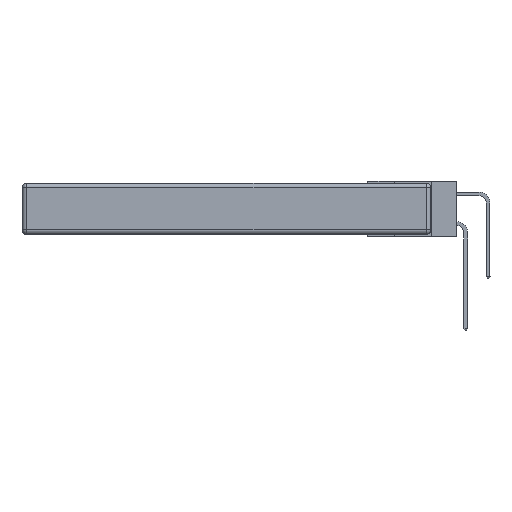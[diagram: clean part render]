
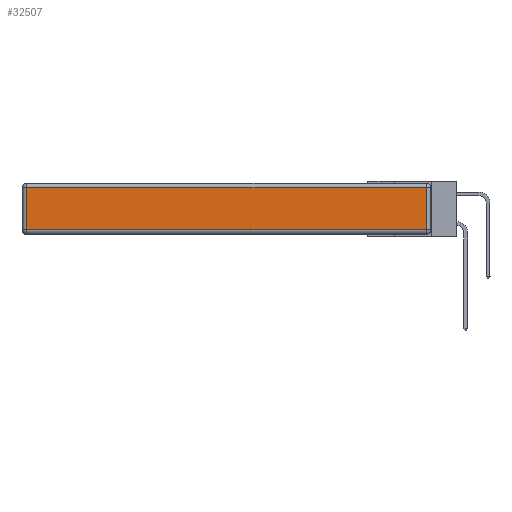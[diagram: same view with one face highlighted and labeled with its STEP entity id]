
A CAD part, left-side view. The second image highlights one B-rep face of the part: STEP entity #32507.
In plain terms, the highlighted planar face has unit normal (-1, 0, 0).
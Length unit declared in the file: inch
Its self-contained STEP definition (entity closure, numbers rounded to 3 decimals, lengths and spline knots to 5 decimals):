
#805 = CARTESIAN_POINT ( 'NONE',  ( 0., 2.72, -0.313 ) ) ;
#832 = DIRECTION ( 'NONE',  ( 0., 1., 0. ) ) ;
#5177 = PLANE ( 'NONE',  #20323 ) ;
#7078 = VECTOR ( 'NONE', #30993, 39.37008 ) ;
#7398 = FACE_OUTER_BOUND ( 'NONE', #22321, .T. ) ;
#8135 = DIRECTION ( 'NONE',  ( -1., 0., 0. ) ) ;
#10450 = VERTEX_POINT ( 'NONE', #32990 ) ;
#11434 = VECTOR ( 'NONE', #26426, 39.37008 ) ;
#12628 = ORIENTED_EDGE ( 'NONE', *, *, #14009, .T. ) ;
#13937 = LINE ( 'NONE', #31110, #7078 ) ;
#14009 = EDGE_CURVE ( 'NONE', #36515, #34124, #23431, .T. ) ;
#15105 = CARTESIAN_POINT ( 'NONE',  ( 0., 2.72, -0.343 ) ) ;
#16077 = LINE ( 'NONE', #18349, #26584 ) ;
#16870 = ORIENTED_EDGE ( 'NONE', *, *, #22963, .T. ) ;
#17742 = CARTESIAN_POINT ( 'NONE',  ( 0., 0., -0.313 ) ) ;
#18051 = EDGE_CURVE ( 'NONE', #35482, #36515, #16077, .T. ) ;
#18349 = CARTESIAN_POINT ( 'NONE',  ( 0., 2.75, -0.03 ) ) ;
#19159 = LINE ( 'NONE', #17742, #11434 ) ;
#20323 = AXIS2_PLACEMENT_3D ( 'NONE', #25587, #8135, #28545 ) ;
#20985 = DIRECTION ( 'NONE',  ( 0., 0., -1. ) ) ;
#21363 = ORIENTED_EDGE ( 'NONE', *, *, #18051, .T. ) ;
#22321 = EDGE_LOOP ( 'NONE', ( #23688, #16870, #21363, #12628 ) ) ;
#22963 = EDGE_CURVE ( 'NONE', #10450, #35482, #13937, .T. ) ;
#22995 = VECTOR ( 'NONE', #20985, 39.37008 ) ;
#23431 = LINE ( 'NONE', #15105, #22995 ) ;
#23688 = ORIENTED_EDGE ( 'NONE', *, *, #28860, .T. ) ;
#25587 = CARTESIAN_POINT ( 'NONE',  ( 0., 0., -0.343 ) ) ;
#26426 = DIRECTION ( 'NONE',  ( 0., -1., 0. ) ) ;
#26584 = VECTOR ( 'NONE', #832, 39.37008 ) ;
#27303 = CARTESIAN_POINT ( 'NONE',  ( 0., 0.03, -0.03 ) ) ;
#28545 = DIRECTION ( 'NONE',  ( 0., 0., 1. ) ) ;
#28860 = EDGE_CURVE ( 'NONE', #34124, #10450, #19159, .T. ) ;
#30993 = DIRECTION ( 'NONE',  ( 0., 0., 1. ) ) ;
#31110 = CARTESIAN_POINT ( 'NONE',  ( 0., 0.03, -0.343 ) ) ;
#32507 = ADVANCED_FACE ( 'NONE', ( #7398 ), #5177, .T. ) ;
#32990 = CARTESIAN_POINT ( 'NONE',  ( 0., 0.03, -0.313 ) ) ;
#34124 = VERTEX_POINT ( 'NONE', #805 ) ;
#35482 = VERTEX_POINT ( 'NONE', #27303 ) ;
#36515 = VERTEX_POINT ( 'NONE', #37537 ) ;
#37537 = CARTESIAN_POINT ( 'NONE',  ( 0., 2.72, -0.03 ) ) ;
